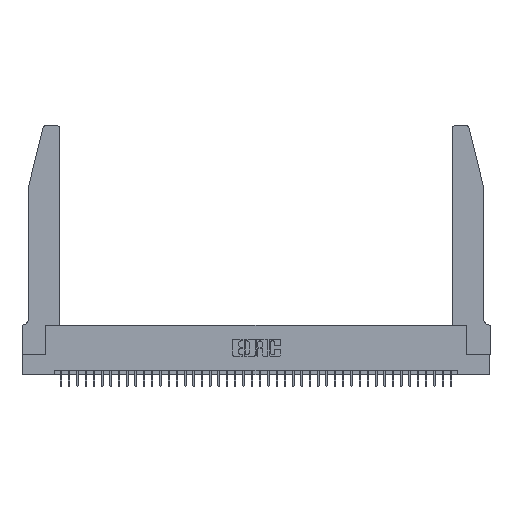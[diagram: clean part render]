
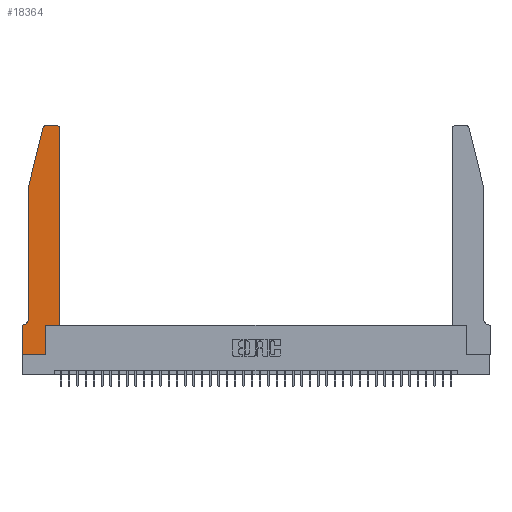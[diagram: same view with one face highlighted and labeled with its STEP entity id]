
A CAD part, top view. The second image highlights one B-rep face of the part: STEP entity #18364.
In plain terms, the highlighted planar face has unit normal (0, 0, 1).
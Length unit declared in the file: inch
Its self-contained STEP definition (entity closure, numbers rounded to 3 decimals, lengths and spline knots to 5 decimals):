
#680 = ORIENTED_EDGE ( 'NONE', *, *, #32808, .T. ) ;
#1230 = CARTESIAN_POINT ( 'NONE',  ( 0.284, 2.75, 0.37 ) ) ;
#1438 = DIRECTION ( 'NONE',  ( 0., 0., 1. ) ) ;
#1723 = VECTOR ( 'NONE', #10636, 39.37008 ) ;
#1884 = CARTESIAN_POINT ( 'NONE',  ( 0.4505, 0.35, 0.37 ) ) ;
#2125 = ORIENTED_EDGE ( 'NONE', *, *, #18502, .T. ) ;
#2406 = AXIS2_PLACEMENT_3D ( 'NONE', #13076, #6575, #9923 ) ;
#2969 = VERTEX_POINT ( 'NONE', #38313 ) ;
#3562 = DIRECTION ( 'NONE',  ( -1., 0., 0. ) ) ;
#3783 = VERTEX_POINT ( 'NONE', #31182 ) ;
#4110 = EDGE_CURVE ( 'NONE', #18359, #31875, #27144, .T. ) ;
#4531 = FACE_OUTER_BOUND ( 'NONE', #37421, .T. ) ;
#5032 = DIRECTION ( 'NONE',  ( 1., 0., 0. ) ) ;
#5259 = VERTEX_POINT ( 'NONE', #25752 ) ;
#5426 = VERTEX_POINT ( 'NONE', #1230 ) ;
#5964 = ORIENTED_EDGE ( 'NONE', *, *, #4110, .T. ) ;
#6549 = CARTESIAN_POINT ( 'NONE',  ( 0.4205, 2.75, 0.37 ) ) ;
#6575 = DIRECTION ( 'NONE',  ( 0., 0., -1. ) ) ;
#6637 = EDGE_CURVE ( 'NONE', #5426, #9980, #33427, .T. ) ;
#6655 = CARTESIAN_POINT ( 'NONE',  ( 0., 0., 0.37 ) ) ;
#7024 = ORIENTED_EDGE ( 'NONE', *, *, #20594, .T. ) ;
#7615 = ORIENTED_EDGE ( 'NONE', *, *, #33396, .T. ) ;
#7661 = ORIENTED_EDGE ( 'NONE', *, *, #16375, .T. ) ;
#9059 = CARTESIAN_POINT ( 'NONE',  ( 0.2865, 0., 0.37 ) ) ;
#9923 = DIRECTION ( 'NONE',  ( -1., 0., 0. ) ) ;
#9980 = VERTEX_POINT ( 'NONE', #39728 ) ;
#10636 = DIRECTION ( 'NONE',  ( -0.239, -0.971, 0. ) ) ;
#12253 = VECTOR ( 'NONE', #32774, 39.37008 ) ;
#12424 = VECTOR ( 'NONE', #36335, 39.37008 ) ;
#12513 = AXIS2_PLACEMENT_3D ( 'NONE', #40192, #20573, #17391 ) ;
#12832 = DIRECTION ( 'NONE',  ( 0., 1., 0. ) ) ;
#13076 = CARTESIAN_POINT ( 'NONE',  ( 0.0055, 0.42, 0.37 ) ) ;
#14375 = DIRECTION ( 'NONE',  ( 1., 0., 0. ) ) ;
#14591 = DIRECTION ( 'NONE',  ( 0., 0., 1. ) ) ;
#15386 = CARTESIAN_POINT ( 'NONE',  ( 0.2865, 0.35, 0.37 ) ) ;
#15811 = LINE ( 'NONE', #41166, #17780 ) ;
#16328 = VERTEX_POINT ( 'NONE', #9059 ) ;
#16375 = EDGE_CURVE ( 'NONE', #2969, #5259, #15811, .T. ) ;
#16507 = VECTOR ( 'NONE', #12832, 39.37008 ) ;
#17368 = CARTESIAN_POINT ( 'NONE',  ( 0.2865, 0.35, 0.37 ) ) ;
#17391 = DIRECTION ( 'NONE',  ( 1., 0., 0. ) ) ;
#17519 = EDGE_CURVE ( 'NONE', #16328, #38016, #21567, .T. ) ;
#17780 = VECTOR ( 'NONE', #25543, 39.37008 ) ;
#18359 = VERTEX_POINT ( 'NONE', #39978 ) ;
#18364 = ADVANCED_FACE ( 'NONE', ( #4531 ), #20779, .T. ) ;
#18502 = EDGE_CURVE ( 'NONE', #9980, #2969, #36196, .T. ) ;
#19538 = DIRECTION ( 'NONE',  ( 0., -1., 0. ) ) ;
#19772 = VECTOR ( 'NONE', #19538, 39.37008 ) ;
#19820 = VECTOR ( 'NONE', #21215, 39.37008 ) ;
#20573 = DIRECTION ( 'NONE',  ( 0., 0., 1. ) ) ;
#20594 = EDGE_CURVE ( 'NONE', #5259, #24101, #26668, .T. ) ;
#20779 = PLANE ( 'NONE',  #12513 ) ;
#21215 = DIRECTION ( 'NONE',  ( 0., 1., 0. ) ) ;
#21464 = EDGE_CURVE ( 'NONE', #31875, #34777, #24722, .T. ) ;
#21496 = VERTEX_POINT ( 'NONE', #30043 ) ;
#21567 = LINE ( 'NONE', #15386, #16507 ) ;
#21819 = LINE ( 'NONE', #34700, #12253 ) ;
#23064 = CARTESIAN_POINT ( 'NONE',  ( 0., 0., 0.37 ) ) ;
#23319 = EDGE_CURVE ( 'NONE', #34777, #5426, #33303, .T. ) ;
#24032 = AXIS2_PLACEMENT_3D ( 'NONE', #33732, #1438, #5032 ) ;
#24101 = VERTEX_POINT ( 'NONE', #38516 ) ;
#24722 = CIRCLE ( 'NONE', #41597, 0.03 ) ;
#25543 = DIRECTION ( 'NONE',  ( 0., -1., 0. ) ) ;
#25572 = EDGE_CURVE ( 'NONE', #21496, #3783, #36185, .T. ) ;
#25752 = CARTESIAN_POINT ( 'NONE',  ( 0.0755, 0.42, 0.37 ) ) ;
#25809 = LINE ( 'NONE', #23064, #12424 ) ;
#26366 = CARTESIAN_POINT ( 'NONE',  ( 0.2605, 2.75, 0.37 ) ) ;
#26542 = ORIENTED_EDGE ( 'NONE', *, *, #17519, .T. ) ;
#26668 = CIRCLE ( 'NONE', #2406, 0.07 ) ;
#26699 = CARTESIAN_POINT ( 'NONE',  ( 0.0755, 2., 0.37 ) ) ;
#27030 = EDGE_CURVE ( 'NONE', #3783, #16328, #25809, .T. ) ;
#27144 = LINE ( 'NONE', #27761, #19820 ) ;
#27487 = CARTESIAN_POINT ( 'NONE',  ( 0.4205, 2.72, 0.37 ) ) ;
#27761 = CARTESIAN_POINT ( 'NONE',  ( 0.4505, 0.35, 0.37 ) ) ;
#28482 = DIRECTION ( 'NONE',  ( 1., 0., 0. ) ) ;
#29620 = VECTOR ( 'NONE', #3562, 39.37008 ) ;
#29622 = ORIENTED_EDGE ( 'NONE', *, *, #6637, .T. ) ;
#30043 = CARTESIAN_POINT ( 'NONE',  ( 0., 0.35, 0.37 ) ) ;
#31182 = CARTESIAN_POINT ( 'NONE',  ( 0., 0., 0.37 ) ) ;
#31875 = VERTEX_POINT ( 'NONE', #40780 ) ;
#32301 = ORIENTED_EDGE ( 'NONE', *, *, #21464, .T. ) ;
#32774 = DIRECTION ( 'NONE',  ( -1., 0., 0. ) ) ;
#32808 = EDGE_CURVE ( 'NONE', #24101, #21496, #21819, .T. ) ;
#33303 = LINE ( 'NONE', #26366, #29620 ) ;
#33396 = EDGE_CURVE ( 'NONE', #38016, #18359, #40520, .T. ) ;
#33427 = CIRCLE ( 'NONE', #24032, 0.03 ) ;
#33732 = CARTESIAN_POINT ( 'NONE',  ( 0.284, 2.72, 0.37 ) ) ;
#34700 = CARTESIAN_POINT ( 'NONE',  ( 0.0755, 0.35, 0.37 ) ) ;
#34777 = VERTEX_POINT ( 'NONE', #6549 ) ;
#35874 = VECTOR ( 'NONE', #28482, 39.37008 ) ;
#36185 = LINE ( 'NONE', #6655, #19772 ) ;
#36196 = LINE ( 'NONE', #26699, #1723 ) ;
#36335 = DIRECTION ( 'NONE',  ( 1., 0., 0. ) ) ;
#37421 = EDGE_LOOP ( 'NONE', ( #40170, #29622, #2125, #7661, #7024, #680, #39915, #41245, #26542, #7615, #5964, #32301 ) ) ;
#38016 = VERTEX_POINT ( 'NONE', #17368 ) ;
#38313 = CARTESIAN_POINT ( 'NONE',  ( 0.0755, 2., 0.37 ) ) ;
#38516 = CARTESIAN_POINT ( 'NONE',  ( 0.0055, 0.35, 0.37 ) ) ;
#39728 = CARTESIAN_POINT ( 'NONE',  ( 0.25487, 2.72718, 0.37 ) ) ;
#39915 = ORIENTED_EDGE ( 'NONE', *, *, #25572, .T. ) ;
#39978 = CARTESIAN_POINT ( 'NONE',  ( 0.4505, 0.35, 0.37 ) ) ;
#40170 = ORIENTED_EDGE ( 'NONE', *, *, #23319, .T. ) ;
#40192 = CARTESIAN_POINT ( 'NONE',  ( 0., 0.35, 0.37 ) ) ;
#40520 = LINE ( 'NONE', #1884, #35874 ) ;
#40780 = CARTESIAN_POINT ( 'NONE',  ( 0.4505, 2.72, 0.37 ) ) ;
#41166 = CARTESIAN_POINT ( 'NONE',  ( 0.0755, 2., 0.37 ) ) ;
#41245 = ORIENTED_EDGE ( 'NONE', *, *, #27030, .T. ) ;
#41597 = AXIS2_PLACEMENT_3D ( 'NONE', #27487, #14591, #14375 ) ;
